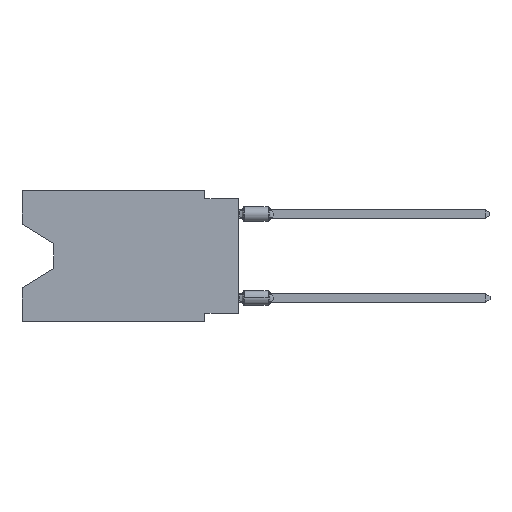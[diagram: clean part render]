
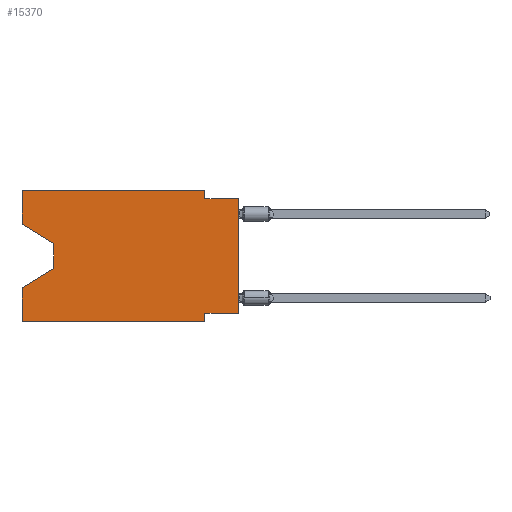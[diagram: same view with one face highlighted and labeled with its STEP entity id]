
A CAD part, left-side view. The second image highlights one B-rep face of the part: STEP entity #15370.
In plain terms, the highlighted planar face has unit normal (-1, 0, 0).
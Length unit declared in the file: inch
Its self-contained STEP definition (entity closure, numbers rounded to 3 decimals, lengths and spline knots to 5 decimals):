
#2435 = LINE ( 'NONE', #17133, #51645 ) ;
#2607 = CARTESIAN_POINT ( 'NONE',  ( 0., 0.645, 0. ) ) ;
#2945 = CARTESIAN_POINT ( 'NONE',  ( 0., 0.645, -0.39 ) ) ;
#3523 = LINE ( 'NONE', #2607, #44409 ) ;
#4541 = VECTOR ( 'NONE', #52332, 39.37008 ) ;
#4588 = DIRECTION ( 'NONE',  ( 0., 0., -1. ) ) ;
#5267 = VERTEX_POINT ( 'NONE', #8318 ) ;
#5497 = LINE ( 'NONE', #38298, #10340 ) ;
#6428 = VECTOR ( 'NONE', #40627, 39.37008 ) ;
#8318 = CARTESIAN_POINT ( 'NONE',  ( 0., 0.55, -0.232 ) ) ;
#8491 = DIRECTION ( 'NONE',  ( 0., 1., 0. ) ) ;
#9474 = CARTESIAN_POINT ( 'NONE',  ( 0., 0.645, 0. ) ) ;
#10229 = EDGE_CURVE ( 'NONE', #33473, #21364, #32073, .T. ) ;
#10340 = VECTOR ( 'NONE', #42006, 39.37008 ) ;
#10471 = VERTEX_POINT ( 'NONE', #56596 ) ;
#11624 = LINE ( 'NONE', #25411, #42742 ) ;
#11709 = EDGE_LOOP ( 'NONE', ( #20482, #21634, #30416, #24506, #21967, #14576, #58405, #58630, #11817, #41861, #37145, #46839 ) ) ;
#11817 = ORIENTED_EDGE ( 'NONE', *, *, #43429, .F. ) ;
#12678 = EDGE_CURVE ( 'NONE', #42005, #24400, #11624, .T. ) ;
#13003 = CARTESIAN_POINT ( 'NONE',  ( 0., 0.1, 0. ) ) ;
#13385 = LINE ( 'NONE', #40708, #29834 ) ;
#14056 = DIRECTION ( 'NONE',  ( 0., 0., -1. ) ) ;
#14095 = VECTOR ( 'NONE', #4588, 39.37008 ) ;
#14522 = CARTESIAN_POINT ( 'NONE',  ( 0., 0.645, 0. ) ) ;
#14576 = ORIENTED_EDGE ( 'NONE', *, *, #26212, .F. ) ;
#15370 = ADVANCED_FACE ( 'NONE', ( #22655 ), #32170, .F. ) ;
#15807 = EDGE_CURVE ( 'NONE', #23879, #53796, #13385, .T. ) ;
#16531 = DIRECTION ( 'NONE',  ( 0., 0., -1. ) ) ;
#17133 = CARTESIAN_POINT ( 'NONE',  ( 0., 0.1, 0. ) ) ;
#20482 = ORIENTED_EDGE ( 'NONE', *, *, #60446, .T. ) ;
#21364 = VERTEX_POINT ( 'NONE', #43619 ) ;
#21430 = DIRECTION ( 'NONE',  ( 0., -1., 0. ) ) ;
#21634 = ORIENTED_EDGE ( 'NONE', *, *, #23422, .T. ) ;
#21775 = LINE ( 'NONE', #35290, #45195 ) ;
#21967 = ORIENTED_EDGE ( 'NONE', *, *, #10229, .T. ) ;
#22655 = FACE_OUTER_BOUND ( 'NONE', #11709, .T. ) ;
#22809 = LINE ( 'NONE', #37228, #6428 ) ;
#23269 = DIRECTION ( 'NONE',  ( 1., 0., 0. ) ) ;
#23422 = EDGE_CURVE ( 'NONE', #10471, #5267, #27862, .T. ) ;
#23879 = VERTEX_POINT ( 'NONE', #31045 ) ;
#24400 = VERTEX_POINT ( 'NONE', #13003 ) ;
#24506 = ORIENTED_EDGE ( 'NONE', *, *, #40615, .F. ) ;
#25411 = CARTESIAN_POINT ( 'NONE',  ( 0., 0.645, 0. ) ) ;
#26212 = EDGE_CURVE ( 'NONE', #53796, #21364, #21775, .T. ) ;
#26830 = AXIS2_PLACEMENT_3D ( 'NONE', #9474, #23269, #14056 ) ;
#27052 = CARTESIAN_POINT ( 'NONE',  ( 0., 0., -0.025 ) ) ;
#27797 = VERTEX_POINT ( 'NONE', #57339 ) ;
#27862 = LINE ( 'NONE', #46598, #14095 ) ;
#29521 = VERTEX_POINT ( 'NONE', #50701 ) ;
#29834 = VECTOR ( 'NONE', #8491, 39.37008 ) ;
#30416 = ORIENTED_EDGE ( 'NONE', *, *, #37773, .T. ) ;
#31045 = CARTESIAN_POINT ( 'NONE',  ( 0., 0., -0.365 ) ) ;
#32073 = LINE ( 'NONE', #2945, #38897 ) ;
#32170 = PLANE ( 'NONE',  #26830 ) ;
#32863 = VERTEX_POINT ( 'NONE', #56315 ) ;
#33473 = VERTEX_POINT ( 'NONE', #45768 ) ;
#35290 = CARTESIAN_POINT ( 'NONE',  ( 0., 0.1, -0.39 ) ) ;
#37145 = ORIENTED_EDGE ( 'NONE', *, *, #12678, .F. ) ;
#37228 = CARTESIAN_POINT ( 'NONE',  ( 0., 0.645, 0. ) ) ;
#37773 = EDGE_CURVE ( 'NONE', #5267, #29521, #52023, .T. ) ;
#38298 = CARTESIAN_POINT ( 'NONE',  ( 0., 0.645, -0.10025 ) ) ;
#38897 = VECTOR ( 'NONE', #45887, 39.37008 ) ;
#39821 = VECTOR ( 'NONE', #55892, 39.37008 ) ;
#40615 = EDGE_CURVE ( 'NONE', #33473, #29521, #22809, .T. ) ;
#40627 = DIRECTION ( 'NONE',  ( 0., 0., 1. ) ) ;
#40708 = CARTESIAN_POINT ( 'NONE',  ( 0., 0., -0.365 ) ) ;
#41861 = ORIENTED_EDGE ( 'NONE', *, *, #44234, .F. ) ;
#42005 = VERTEX_POINT ( 'NONE', #14522 ) ;
#42006 = DIRECTION ( 'NONE',  ( 0., -0.855, -0.519 ) ) ;
#42544 = CARTESIAN_POINT ( 'NONE',  ( 0., 0.55, -0.232 ) ) ;
#42733 = CARTESIAN_POINT ( 'NONE',  ( 0., 0.1, -0.365 ) ) ;
#42742 = VECTOR ( 'NONE', #21430, 39.37008 ) ;
#43429 = EDGE_CURVE ( 'NONE', #27797, #46438, #46397, .T. ) ;
#43619 = CARTESIAN_POINT ( 'NONE',  ( 0., 0.1, -0.39 ) ) ;
#44234 = EDGE_CURVE ( 'NONE', #24400, #27797, #2435, .T. ) ;
#44409 = VECTOR ( 'NONE', #45216, 39.37008 ) ;
#44498 = DIRECTION ( 'NONE',  ( 0., 0., -1. ) ) ;
#45195 = VECTOR ( 'NONE', #44498, 39.37008 ) ;
#45216 = DIRECTION ( 'NONE',  ( 0., 0., 1. ) ) ;
#45768 = CARTESIAN_POINT ( 'NONE',  ( 0., 0.645, -0.39 ) ) ;
#45887 = DIRECTION ( 'NONE',  ( 0., -1., 0. ) ) ;
#46397 = LINE ( 'NONE', #27052, #39821 ) ;
#46438 = VERTEX_POINT ( 'NONE', #57678 ) ;
#46598 = CARTESIAN_POINT ( 'NONE',  ( 0., 0.55, -0.158 ) ) ;
#46839 = ORIENTED_EDGE ( 'NONE', *, *, #57585, .F. ) ;
#47792 = DIRECTION ( 'NONE',  ( 0., 0., 1. ) ) ;
#49361 = EDGE_CURVE ( 'NONE', #23879, #46438, #52973, .T. ) ;
#50701 = CARTESIAN_POINT ( 'NONE',  ( 0., 0.645, -0.28975 ) ) ;
#51645 = VECTOR ( 'NONE', #16531, 39.37008 ) ;
#52023 = LINE ( 'NONE', #42544, #4541 ) ;
#52065 = CARTESIAN_POINT ( 'NONE',  ( 0., 0., 0. ) ) ;
#52332 = DIRECTION ( 'NONE',  ( 0., 0.855, -0.519 ) ) ;
#52973 = LINE ( 'NONE', #52065, #55658 ) ;
#53796 = VERTEX_POINT ( 'NONE', #42733 ) ;
#55658 = VECTOR ( 'NONE', #47792, 39.37008 ) ;
#55892 = DIRECTION ( 'NONE',  ( 0., -1., 0. ) ) ;
#56315 = CARTESIAN_POINT ( 'NONE',  ( 0., 0.645, -0.10025 ) ) ;
#56596 = CARTESIAN_POINT ( 'NONE',  ( 0., 0.55, -0.158 ) ) ;
#57339 = CARTESIAN_POINT ( 'NONE',  ( 0., 0.1, -0.025 ) ) ;
#57585 = EDGE_CURVE ( 'NONE', #32863, #42005, #3523, .T. ) ;
#57678 = CARTESIAN_POINT ( 'NONE',  ( 0., 0., -0.025 ) ) ;
#58405 = ORIENTED_EDGE ( 'NONE', *, *, #15807, .F. ) ;
#58630 = ORIENTED_EDGE ( 'NONE', *, *, #49361, .T. ) ;
#60446 = EDGE_CURVE ( 'NONE', #32863, #10471, #5497, .T. ) ;
